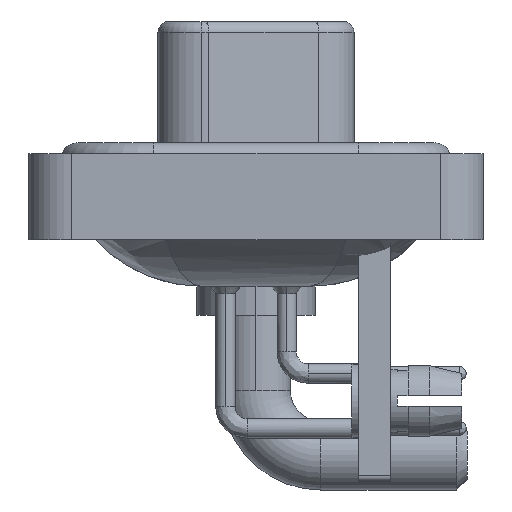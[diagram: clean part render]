
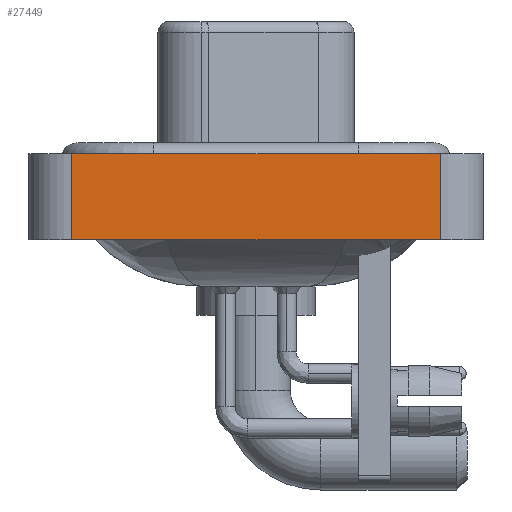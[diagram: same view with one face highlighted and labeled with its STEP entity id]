
A CAD part, left-side view. The second image highlights one B-rep face of the part: STEP entity #27449.
In plain terms, the highlighted planar face has unit normal (-1, 0, 0).
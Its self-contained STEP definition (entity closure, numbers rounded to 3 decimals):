
#2265 = EDGE_CURVE ( 'NONE', #28364, #30733, #27962, .T. ) ;
#2744 = CARTESIAN_POINT ( 'NONE',  ( -7.35, 8.55, 0.4 ) ) ;
#4212 = VERTEX_POINT ( 'NONE', #16954 ) ;
#4279 = VECTOR ( 'NONE', #10363, 1000. ) ;
#5852 = DIRECTION ( 'NONE',  ( 0., 0., 1. ) ) ;
#6985 = VECTOR ( 'NONE', #19503, 1000. ) ;
#9177 = CARTESIAN_POINT ( 'NONE',  ( -7.35, -8.55, -3.6 ) ) ;
#9633 = DIRECTION ( 'NONE',  ( 0., -1., 0. ) ) ;
#9655 = LINE ( 'NONE', #9177, #6985 ) ;
#10363 = DIRECTION ( 'NONE',  ( 0., 0., 1. ) ) ;
#11075 = ORIENTED_EDGE ( 'NONE', *, *, #21605, .T. ) ;
#11522 = VECTOR ( 'NONE', #9633, 1000. ) ;
#11774 = PLANE ( 'NONE',  #30905 ) ;
#12015 = CARTESIAN_POINT ( 'NONE',  ( -7.35, -8.55, -3.6 ) ) ;
#12310 = CARTESIAN_POINT ( 'NONE',  ( -7.35, -8.55, 0.4 ) ) ;
#12927 = EDGE_LOOP ( 'NONE', ( #22096, #14174, #20434, #11075 ) ) ;
#14142 = CARTESIAN_POINT ( 'NONE',  ( -7.35, -8.55, 0.4 ) ) ;
#14174 = ORIENTED_EDGE ( 'NONE', *, *, #20283, .F. ) ;
#15206 = LINE ( 'NONE', #27944, #4279 ) ;
#16447 = DIRECTION ( 'NONE',  ( -1., 0., 0. ) ) ;
#16954 = CARTESIAN_POINT ( 'NONE',  ( -7.35, 8.55, -3.6 ) ) ;
#19503 = DIRECTION ( 'NONE',  ( 0., -1., 0. ) ) ;
#19727 = EDGE_CURVE ( 'NONE', #4212, #27216, #15206, .T. ) ;
#20283 = EDGE_CURVE ( 'NONE', #27216, #30733, #23682, .T. ) ;
#20434 = ORIENTED_EDGE ( 'NONE', *, *, #19727, .F. ) ;
#21605 = EDGE_CURVE ( 'NONE', #4212, #28364, #9655, .T. ) ;
#21620 = CARTESIAN_POINT ( 'NONE',  ( -7.35, -8.55, -3.6 ) ) ;
#22096 = ORIENTED_EDGE ( 'NONE', *, *, #2265, .T. ) ;
#22251 = VECTOR ( 'NONE', #5852, 1000. ) ;
#23682 = LINE ( 'NONE', #14142, #11522 ) ;
#24045 = FACE_OUTER_BOUND ( 'NONE', #12927, .T. ) ;
#27216 = VERTEX_POINT ( 'NONE', #2744 ) ;
#27449 = ADVANCED_FACE ( 'NONE', ( #24045 ), #11774, .T. ) ;
#27944 = CARTESIAN_POINT ( 'NONE',  ( -7.35, 8.55, -3.6 ) ) ;
#27962 = LINE ( 'NONE', #30576, #22251 ) ;
#28364 = VERTEX_POINT ( 'NONE', #12015 ) ;
#30576 = CARTESIAN_POINT ( 'NONE',  ( -7.35, -8.55, -3.6 ) ) ;
#30733 = VERTEX_POINT ( 'NONE', #12310 ) ;
#30905 = AXIS2_PLACEMENT_3D ( 'NONE', #21620, #16447, #31481 ) ;
#31481 = DIRECTION ( 'NONE',  ( 0., 0., 1. ) ) ;
